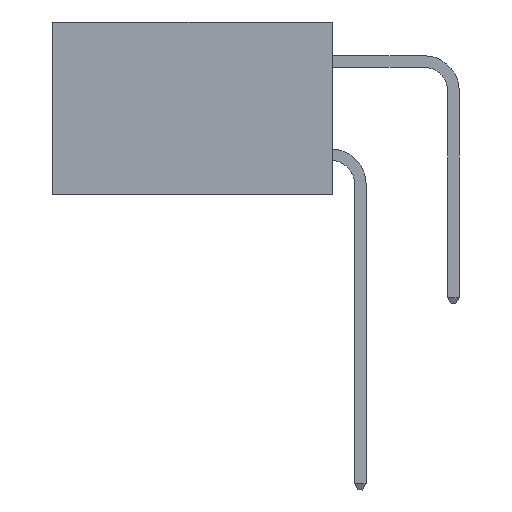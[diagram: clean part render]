
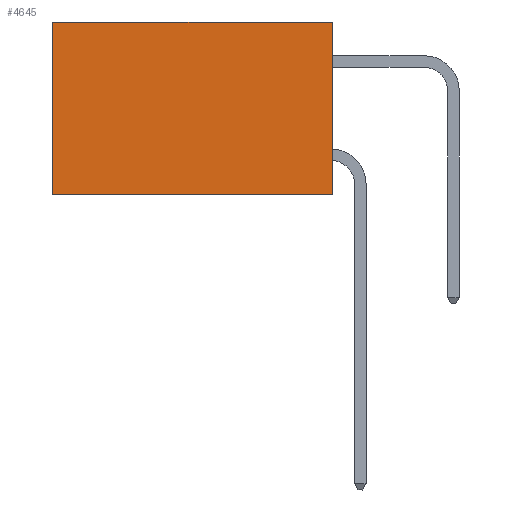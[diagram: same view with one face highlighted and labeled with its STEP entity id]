
A CAD part, left-side view. The second image highlights one B-rep face of the part: STEP entity #4645.
In plain terms, the highlighted planar face has unit normal (-1, 0, 0).
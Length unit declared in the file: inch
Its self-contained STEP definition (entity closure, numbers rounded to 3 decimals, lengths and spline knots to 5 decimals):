
#658 = VECTOR ( 'NONE', #7208, 39.37008 ) ;
#1912 = EDGE_CURVE ( 'NONE', #5180, #5827, #4173, .T. ) ;
#1936 = LINE ( 'NONE', #14938, #5703 ) ;
#2349 = EDGE_CURVE ( 'NONE', #5180, #15344, #9955, .T. ) ;
#2598 = VECTOR ( 'NONE', #4414, 39.37008 ) ;
#2971 = ORIENTED_EDGE ( 'NONE', *, *, #1912, .F. ) ;
#2984 = EDGE_CURVE ( 'NONE', #15344, #12502, #10192, .T. ) ;
#3699 = CARTESIAN_POINT ( 'NONE',  ( 0.298, 0.6, -0.37 ) ) ;
#4173 = LINE ( 'NONE', #14665, #658 ) ;
#4414 = DIRECTION ( 'NONE',  ( 0., 0., -1. ) ) ;
#4465 = ORIENTED_EDGE ( 'NONE', *, *, #2349, .T. ) ;
#4645 = ADVANCED_FACE ( 'NONE', ( #17049 ), #10834, .F. ) ;
#4657 = CARTESIAN_POINT ( 'NONE',  ( 0.298, 0.6, 0. ) ) ;
#5180 = VERTEX_POINT ( 'NONE', #8529 ) ;
#5703 = VECTOR ( 'NONE', #7053, 39.37008 ) ;
#5827 = VERTEX_POINT ( 'NONE', #15485 ) ;
#7053 = DIRECTION ( 'NONE',  ( 0., 1., 0. ) ) ;
#7208 = DIRECTION ( 'NONE',  ( 0., 0., -1. ) ) ;
#8529 = CARTESIAN_POINT ( 'NONE',  ( 0.298, 0., 0. ) ) ;
#9301 = EDGE_LOOP ( 'NONE', ( #16643, #10391, #2971, #4465 ) ) ;
#9438 = DIRECTION ( 'NONE',  ( 0., 0., -1. ) ) ;
#9955 = LINE ( 'NONE', #10618, #13926 ) ;
#10192 = LINE ( 'NONE', #4657, #2598 ) ;
#10391 = ORIENTED_EDGE ( 'NONE', *, *, #16950, .F. ) ;
#10618 = CARTESIAN_POINT ( 'NONE',  ( 0.298, 0., 0. ) ) ;
#10834 = PLANE ( 'NONE',  #17099 ) ;
#11085 = DIRECTION ( 'NONE',  ( 0., 1., 0. ) ) ;
#11948 = CARTESIAN_POINT ( 'NONE',  ( 0.298, 0., 0. ) ) ;
#12502 = VERTEX_POINT ( 'NONE', #3699 ) ;
#12755 = DIRECTION ( 'NONE',  ( 1., 0., 0. ) ) ;
#13926 = VECTOR ( 'NONE', #11085, 39.37008 ) ;
#14462 = CARTESIAN_POINT ( 'NONE',  ( 0.298, 0.6, 0. ) ) ;
#14665 = CARTESIAN_POINT ( 'NONE',  ( 0.298, 0., 0. ) ) ;
#14938 = CARTESIAN_POINT ( 'NONE',  ( 0.298, 0., -0.37 ) ) ;
#15344 = VERTEX_POINT ( 'NONE', #14462 ) ;
#15485 = CARTESIAN_POINT ( 'NONE',  ( 0.298, 0., -0.37 ) ) ;
#16643 = ORIENTED_EDGE ( 'NONE', *, *, #2984, .T. ) ;
#16950 = EDGE_CURVE ( 'NONE', #5827, #12502, #1936, .T. ) ;
#17049 = FACE_OUTER_BOUND ( 'NONE', #9301, .T. ) ;
#17099 = AXIS2_PLACEMENT_3D ( 'NONE', #11948, #12755, #9438 ) ;
